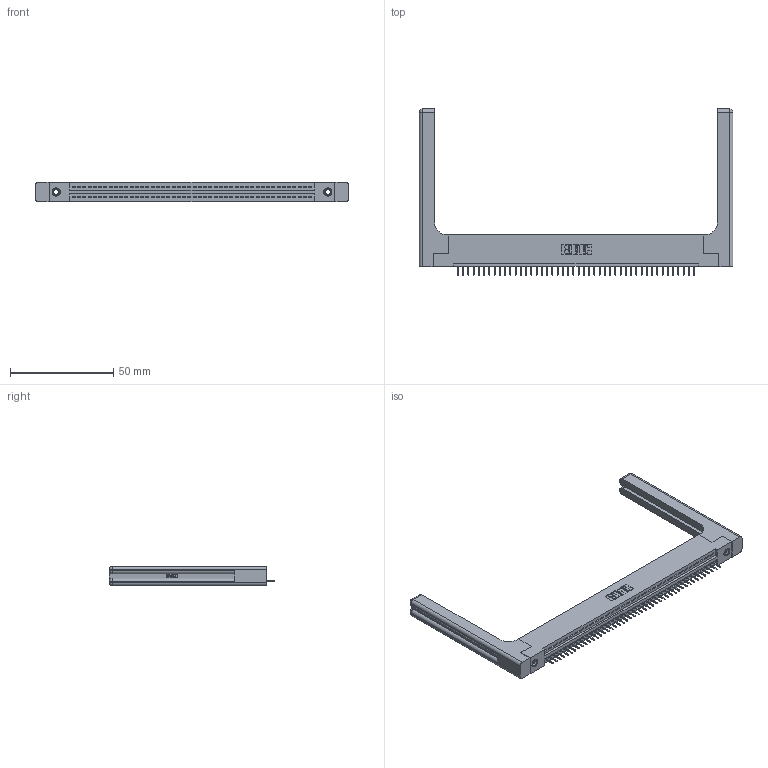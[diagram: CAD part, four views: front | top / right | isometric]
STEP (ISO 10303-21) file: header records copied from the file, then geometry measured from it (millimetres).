
FILE_DESCRIPTION (( 'STEP AP203' ), '1' );
FILE_NAME ('395-046-524-158.STEP', '2019-10-22T20:48:49', ( '' ), ( '' ), 'SwSTEP 2.0', 'SolidWorks 2016', '' );
FILE_SCHEMA (( 'CONFIG_CONTROL_DESIGN' ));
Length unit declared in the file: inch
Products named in the file (5): 345-250-001_345-250-001-102; 345-220-058_345-220-058; 345-292-001_345-293-124; 345 Part_Flush Mounting Lugs - 0.156 Dia-TH; 395-046-524-158
Assembly tree (51 placements, depth 2):
  395-046-524-158
    345 Part_Flush Mounting Lugs - 0.156 Dia-TH
    345-292-001_345-293-124  x46
    345-250-001_345-250-001-102  x2
    345-220-058_345-220-058  x2
Bounding box: 151.87 x 80.31 x 9.4 mm (x, y, z)
Volume: 22780.5 mm3; surface area: 23749.8 mm2
Topology: 51 solids, 51 shells, 3234 faces, 9287 edges, 5986 vertices
Faces by surface type: plane 2344, cylinder 830, bspline 36, cone 12, sphere 8, torus 4
Entity records: 39338 total; most frequent: CARTESIAN_POINT 7783, ORIENTED_EDGE 6560, DIRECTION 5740, EDGE_CURVE 3280, VECTOR 2876, LINE 2876, VERTEX_POINT 2174, AXIS2_PLACEMENT_3D 1432
